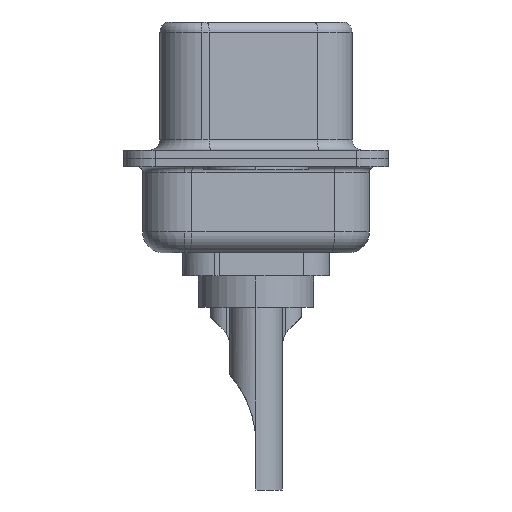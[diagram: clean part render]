
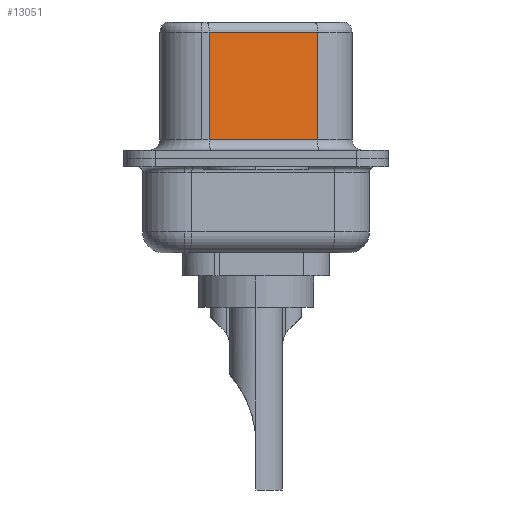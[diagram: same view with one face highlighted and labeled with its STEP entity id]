
A CAD part, left-side view. The second image highlights one B-rep face of the part: STEP entity #13051.
In plain terms, the highlighted planar face has unit normal (-0.985, -0.174, 0).
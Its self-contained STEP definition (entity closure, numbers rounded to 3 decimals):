
#67 = FACE_OUTER_BOUND ( 'NONE', #14732, .T. ) ;
#530 = LINE ( 'NONE', #7077, #6967 ) ;
#1049 = EDGE_CURVE ( 'NONE', #11966, #16636, #530, .T. ) ;
#1518 = ORIENTED_EDGE ( 'NONE', *, *, #5569, .F. ) ;
#1527 = DIRECTION ( 'NONE',  ( -0.174, 0.985, 0. ) ) ;
#2135 = DIRECTION ( 'NONE',  ( 0., 0., -1. ) ) ;
#3656 = EDGE_CURVE ( 'NONE', #14455, #11966, #13247, .T. ) ;
#4687 = AXIS2_PLACEMENT_3D ( 'NONE', #7954, #9250, #1527 ) ;
#4810 = EDGE_CURVE ( 'NONE', #16636, #16373, #9562, .T. ) ;
#5569 = EDGE_CURVE ( 'NONE', #14455, #16373, #9088, .T. ) ;
#5854 = ORIENTED_EDGE ( 'NONE', *, *, #3656, .T. ) ;
#6110 = VECTOR ( 'NONE', #15369, 1000. ) ;
#6360 = VECTOR ( 'NONE', #16720, 1000. ) ;
#6967 = VECTOR ( 'NONE', #13937, 1000. ) ;
#7077 = CARTESIAN_POINT ( 'NONE',  ( 3.675, 2.233, 6.52 ) ) ;
#7954 = CARTESIAN_POINT ( 'NONE',  ( 4.585, -2.927, 6.52 ) ) ;
#8287 = CARTESIAN_POINT ( 'NONE',  ( 3.675, 2.233, 0.9 ) ) ;
#9088 = LINE ( 'NONE', #13748, #15982 ) ;
#9250 = DIRECTION ( 'NONE',  ( 0.985, 0.174, 0. ) ) ;
#9414 = ORIENTED_EDGE ( 'NONE', *, *, #4810, .T. ) ;
#9487 = CARTESIAN_POINT ( 'NONE',  ( 4.585, -2.927, 6.02 ) ) ;
#9562 = LINE ( 'NONE', #11404, #6110 ) ;
#10307 = ORIENTED_EDGE ( 'NONE', *, *, #1049, .T. ) ;
#11404 = CARTESIAN_POINT ( 'NONE',  ( 4.585, -2.927, 0.9 ) ) ;
#11966 = VERTEX_POINT ( 'NONE', #14797 ) ;
#12834 = CARTESIAN_POINT ( 'NONE',  ( 4.585, -2.927, 0.9 ) ) ;
#13051 = ADVANCED_FACE ( 'NONE', ( #67 ), #15713, .F. ) ;
#13247 = LINE ( 'NONE', #9487, #6360 ) ;
#13748 = CARTESIAN_POINT ( 'NONE',  ( 4.585, -2.927, 6.52 ) ) ;
#13937 = DIRECTION ( 'NONE',  ( 0., 0., -1. ) ) ;
#14455 = VERTEX_POINT ( 'NONE', #14934 ) ;
#14732 = EDGE_LOOP ( 'NONE', ( #1518, #5854, #10307, #9414 ) ) ;
#14797 = CARTESIAN_POINT ( 'NONE',  ( 3.675, 2.233, 6.02 ) ) ;
#14934 = CARTESIAN_POINT ( 'NONE',  ( 4.585, -2.927, 6.02 ) ) ;
#15369 = DIRECTION ( 'NONE',  ( 0.174, -0.985, 0. ) ) ;
#15713 = PLANE ( 'NONE',  #4687 ) ;
#15982 = VECTOR ( 'NONE', #2135, 1000. ) ;
#16373 = VERTEX_POINT ( 'NONE', #12834 ) ;
#16636 = VERTEX_POINT ( 'NONE', #8287 ) ;
#16720 = DIRECTION ( 'NONE',  ( -0.174, 0.985, 0. ) ) ;
